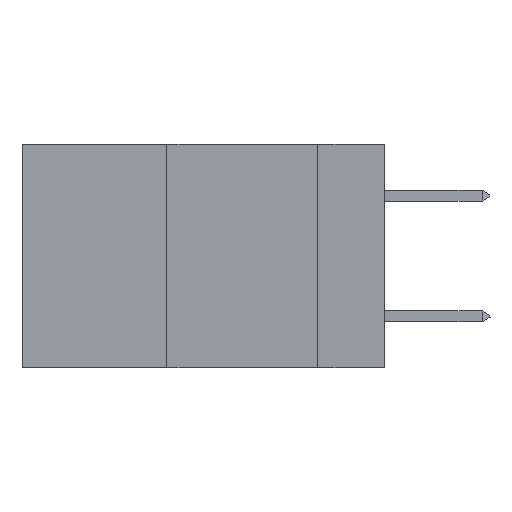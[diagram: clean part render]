
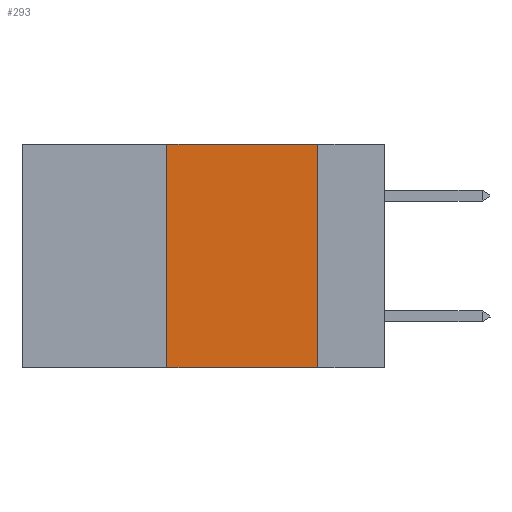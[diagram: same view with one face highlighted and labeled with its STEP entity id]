
A CAD part, left-side view. The second image highlights one B-rep face of the part: STEP entity #293.
In plain terms, the highlighted planar face has unit normal (-1, 0, 0).
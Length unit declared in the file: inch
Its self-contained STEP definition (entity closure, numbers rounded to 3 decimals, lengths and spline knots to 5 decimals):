
#110 = CARTESIAN_POINT ( 'NONE',  ( 0., 0.6, 0. ) ) ;
#293 = ADVANCED_FACE ( 'NONE', ( #25709 ), #10760, .F. ) ;
#860 = DIRECTION ( 'NONE',  ( 0., 0., 1. ) ) ;
#1921 = AXIS2_PLACEMENT_3D ( 'NONE', #110, #25888, #15216 ) ;
#2065 = VERTEX_POINT ( 'NONE', #12097 ) ;
#3102 = LINE ( 'NONE', #19238, #25379 ) ;
#4873 = EDGE_CURVE ( 'NONE', #2065, #13058, #27827, .T. ) ;
#5011 = CARTESIAN_POINT ( 'NONE',  ( 0., 0.6, -0.37 ) ) ;
#5840 = EDGE_CURVE ( 'NONE', #25924, #26576, #3102, .T. ) ;
#6867 = LINE ( 'NONE', #23391, #10578 ) ;
#6919 = ORIENTED_EDGE ( 'NONE', *, *, #4873, .F. ) ;
#9620 = ORIENTED_EDGE ( 'NONE', *, *, #20458, .T. ) ;
#9873 = DIRECTION ( 'NONE',  ( 0., 0., -1. ) ) ;
#10100 = CARTESIAN_POINT ( 'NONE',  ( 0., 0.11, -0.37 ) ) ;
#10578 = VECTOR ( 'NONE', #17070, 39.37008 ) ;
#10760 = PLANE ( 'NONE',  #1921 ) ;
#12097 = CARTESIAN_POINT ( 'NONE',  ( 0., 0.11, 0. ) ) ;
#13058 = VERTEX_POINT ( 'NONE', #10100 ) ;
#13431 = DIRECTION ( 'NONE',  ( 0., -1., 0. ) ) ;
#13640 = CARTESIAN_POINT ( 'NONE',  ( 0., 0.36, 0. ) ) ;
#15216 = DIRECTION ( 'NONE',  ( 0., 0., -1. ) ) ;
#16389 = LINE ( 'NONE', #5011, #17379 ) ;
#17070 = DIRECTION ( 'NONE',  ( 0., -1., 0. ) ) ;
#17379 = VECTOR ( 'NONE', #13431, 39.37008 ) ;
#19238 = CARTESIAN_POINT ( 'NONE',  ( 0., 0.36, 0. ) ) ;
#20093 = ORIENTED_EDGE ( 'NONE', *, *, #20946, .F. ) ;
#20458 = EDGE_CURVE ( 'NONE', #25924, #13058, #16389, .T. ) ;
#20946 = EDGE_CURVE ( 'NONE', #26576, #2065, #6867, .T. ) ;
#21812 = EDGE_LOOP ( 'NONE', ( #6919, #20093, #23319, #9620 ) ) ;
#22981 = CARTESIAN_POINT ( 'NONE',  ( 0., 0.11, 0. ) ) ;
#23039 = VECTOR ( 'NONE', #9873, 39.37008 ) ;
#23319 = ORIENTED_EDGE ( 'NONE', *, *, #5840, .F. ) ;
#23391 = CARTESIAN_POINT ( 'NONE',  ( 0., 0.6, 0. ) ) ;
#24988 = CARTESIAN_POINT ( 'NONE',  ( 0., 0.36, -0.37 ) ) ;
#25379 = VECTOR ( 'NONE', #860, 39.37008 ) ;
#25709 = FACE_OUTER_BOUND ( 'NONE', #21812, .T. ) ;
#25888 = DIRECTION ( 'NONE',  ( 1., 0., 0. ) ) ;
#25924 = VERTEX_POINT ( 'NONE', #24988 ) ;
#26576 = VERTEX_POINT ( 'NONE', #13640 ) ;
#27827 = LINE ( 'NONE', #22981, #23039 ) ;
